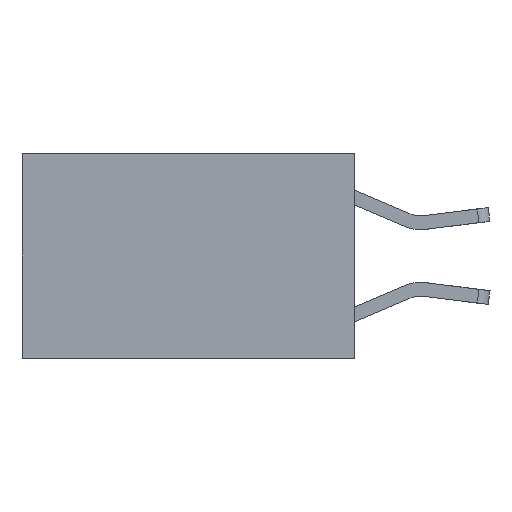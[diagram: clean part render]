
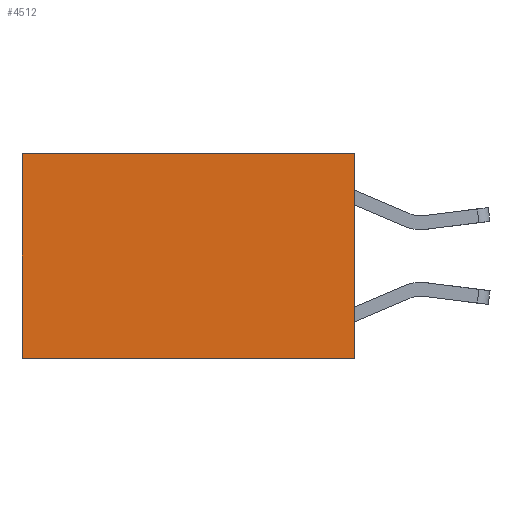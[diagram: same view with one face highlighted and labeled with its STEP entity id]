
A CAD part, left-side view. The second image highlights one B-rep face of the part: STEP entity #4512.
In plain terms, the highlighted planar face has unit normal (-1, 0, 0).
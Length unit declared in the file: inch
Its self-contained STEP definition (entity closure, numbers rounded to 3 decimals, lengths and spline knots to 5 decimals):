
#18 = ORIENTED_EDGE ( 'NONE', *, *, #5536, .T. ) ;
#228 = CARTESIAN_POINT ( 'NONE',  ( 0.2625, 0.6, 0. ) ) ;
#584 = LINE ( 'NONE', #4760, #6921 ) ;
#872 = EDGE_CURVE ( 'NONE', #1110, #1080, #4865, .T. ) ;
#1080 = VERTEX_POINT ( 'NONE', #11007 ) ;
#1110 = VERTEX_POINT ( 'NONE', #4773 ) ;
#2047 = VERTEX_POINT ( 'NONE', #9887 ) ;
#2098 = EDGE_LOOP ( 'NONE', ( #11374, #2246, #4815, #18 ) ) ;
#2246 = ORIENTED_EDGE ( 'NONE', *, *, #6341, .F. ) ;
#2278 = LINE ( 'NONE', #5466, #10746 ) ;
#3330 = DIRECTION ( 'NONE',  ( 1., 0., 0. ) ) ;
#3525 = CARTESIAN_POINT ( 'NONE',  ( 0.2625, 0.6, -0.37 ) ) ;
#3737 = VERTEX_POINT ( 'NONE', #3525 ) ;
#4512 = ADVANCED_FACE ( 'NONE', ( #9357 ), #5253, .F. ) ;
#4760 = CARTESIAN_POINT ( 'NONE',  ( 0.2625, 0., -0.37 ) ) ;
#4773 = CARTESIAN_POINT ( 'NONE',  ( 0.2625, 0., 0. ) ) ;
#4815 = ORIENTED_EDGE ( 'NONE', *, *, #872, .F. ) ;
#4865 = LINE ( 'NONE', #9523, #6948 ) ;
#5129 = DIRECTION ( 'NONE',  ( 0., 0., -1. ) ) ;
#5214 = CARTESIAN_POINT ( 'NONE',  ( 0.2625, 0., 0. ) ) ;
#5253 = PLANE ( 'NONE',  #7438 ) ;
#5466 = CARTESIAN_POINT ( 'NONE',  ( 0.2625, 0., 0. ) ) ;
#5536 = EDGE_CURVE ( 'NONE', #1110, #2047, #2278, .T. ) ;
#5586 = DIRECTION ( 'NONE',  ( 0., 1., 0. ) ) ;
#6126 = LINE ( 'NONE', #228, #6685 ) ;
#6233 = DIRECTION ( 'NONE',  ( 0., 1., 0. ) ) ;
#6341 = EDGE_CURVE ( 'NONE', #1080, #3737, #584, .T. ) ;
#6685 = VECTOR ( 'NONE', #9962, 39.37008 ) ;
#6921 = VECTOR ( 'NONE', #5586, 39.37008 ) ;
#6948 = VECTOR ( 'NONE', #11360, 39.37008 ) ;
#7438 = AXIS2_PLACEMENT_3D ( 'NONE', #5214, #3330, #5129 ) ;
#9357 = FACE_OUTER_BOUND ( 'NONE', #2098, .T. ) ;
#9523 = CARTESIAN_POINT ( 'NONE',  ( 0.2625, 0., 0. ) ) ;
#9887 = CARTESIAN_POINT ( 'NONE',  ( 0.2625, 0.6, 0. ) ) ;
#9962 = DIRECTION ( 'NONE',  ( 0., 0., -1. ) ) ;
#10351 = EDGE_CURVE ( 'NONE', #2047, #3737, #6126, .T. ) ;
#10746 = VECTOR ( 'NONE', #6233, 39.37008 ) ;
#11007 = CARTESIAN_POINT ( 'NONE',  ( 0.2625, 0., -0.37 ) ) ;
#11360 = DIRECTION ( 'NONE',  ( 0., 0., -1. ) ) ;
#11374 = ORIENTED_EDGE ( 'NONE', *, *, #10351, .T. ) ;
